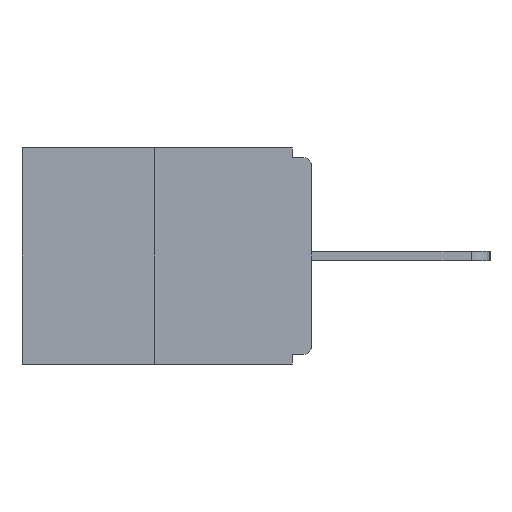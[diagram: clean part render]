
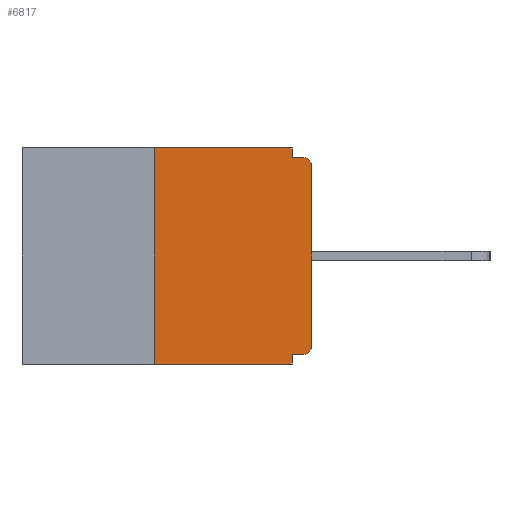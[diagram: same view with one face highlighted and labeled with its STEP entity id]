
A CAD part, left-side view. The second image highlights one B-rep face of the part: STEP entity #6817.
In plain terms, the highlighted planar face has unit normal (-1, 0, 0).
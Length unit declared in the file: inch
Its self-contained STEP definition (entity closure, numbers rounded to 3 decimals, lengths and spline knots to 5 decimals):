
#57 = DIRECTION ( 'NONE',  ( 0., 0., -1. ) ) ;
#111 = DIRECTION ( 'NONE',  ( 1., 0., 0. ) ) ;
#242 = EDGE_CURVE ( 'NONE', #7313, #13654, #5762, .T. ) ;
#287 = DIRECTION ( 'NONE',  ( 0., 0., -1. ) ) ;
#391 = CARTESIAN_POINT ( 'NONE',  ( 0., 0.031, 0. ) ) ;
#524 = DIRECTION ( 'NONE',  ( 0., 0., -1. ) ) ;
#777 = EDGE_CURVE ( 'NONE', #10795, #2583, #3986, .T. ) ;
#800 = DIRECTION ( 'NONE',  ( 0., -1., 0. ) ) ;
#875 = DIRECTION ( 'NONE',  ( -1., 0., 0. ) ) ;
#1165 = CARTESIAN_POINT ( 'NONE',  ( 0., 0.031, -0.328 ) ) ;
#1501 = DIRECTION ( 'NONE',  ( 0., 1., 0. ) ) ;
#1911 = CARTESIAN_POINT ( 'NONE',  ( 0., 0.031, -0.015 ) ) ;
#2117 = CARTESIAN_POINT ( 'NONE',  ( 0., 0.25, 0. ) ) ;
#2214 = CARTESIAN_POINT ( 'NONE',  ( 0., 0.46, 0. ) ) ;
#2464 = LINE ( 'NONE', #10610, #14768 ) ;
#2465 = LINE ( 'NONE', #13090, #2571 ) ;
#2571 = VECTOR ( 'NONE', #14127, 39.37008 ) ;
#2583 = VERTEX_POINT ( 'NONE', #1911 ) ;
#2786 = CARTESIAN_POINT ( 'NONE',  ( 0., 0.015, -0.015 ) ) ;
#2999 = VECTOR ( 'NONE', #13089, 39.37008 ) ;
#3040 = CARTESIAN_POINT ( 'NONE',  ( 0., 0.25, 0. ) ) ;
#3282 = FACE_OUTER_BOUND ( 'NONE', #11460, .T. ) ;
#3318 = AXIS2_PLACEMENT_3D ( 'NONE', #5569, #875, #57 ) ;
#3479 = EDGE_CURVE ( 'NONE', #9759, #9999, #5478, .T. ) ;
#3925 = LINE ( 'NONE', #10988, #14269 ) ;
#3986 = LINE ( 'NONE', #14268, #6601 ) ;
#4028 = DIRECTION ( 'NONE',  ( 0., 0., 1. ) ) ;
#4079 = AXIS2_PLACEMENT_3D ( 'NONE', #2214, #111, #11416 ) ;
#4212 = EDGE_CURVE ( 'NONE', #9239, #10795, #4382, .T. ) ;
#4382 = LINE ( 'NONE', #7358, #14359 ) ;
#4910 = EDGE_CURVE ( 'NONE', #10422, #6604, #2465, .T. ) ;
#5371 = ORIENTED_EDGE ( 'NONE', *, *, #3479, .T. ) ;
#5478 = CIRCLE ( 'NONE', #3318, 0.015 ) ;
#5569 = CARTESIAN_POINT ( 'NONE',  ( 0., 0.015, -0.313 ) ) ;
#5762 = CIRCLE ( 'NONE', #14151, 0.015 ) ;
#5909 = CARTESIAN_POINT ( 'NONE',  ( 0., 0., -0.03 ) ) ;
#6057 = ORIENTED_EDGE ( 'NONE', *, *, #242, .T. ) ;
#6298 = ORIENTED_EDGE ( 'NONE', *, *, #10361, .F. ) ;
#6601 = VECTOR ( 'NONE', #12259, 39.37008 ) ;
#6604 = VERTEX_POINT ( 'NONE', #12731 ) ;
#6817 = ADVANCED_FACE ( 'NONE', ( #3282 ), #7959, .F. ) ;
#6835 = VERTEX_POINT ( 'NONE', #1165 ) ;
#7279 = ORIENTED_EDGE ( 'NONE', *, *, #777, .F. ) ;
#7313 = VERTEX_POINT ( 'NONE', #5909 ) ;
#7329 = ORIENTED_EDGE ( 'NONE', *, *, #11288, .F. ) ;
#7358 = CARTESIAN_POINT ( 'NONE',  ( 0., 0.46, 0. ) ) ;
#7959 = PLANE ( 'NONE',  #4079 ) ;
#8171 = ORIENTED_EDGE ( 'NONE', *, *, #4910, .T. ) ;
#8285 = ORIENTED_EDGE ( 'NONE', *, *, #4212, .F. ) ;
#8504 = LINE ( 'NONE', #10829, #2999 ) ;
#8709 = ORIENTED_EDGE ( 'NONE', *, *, #12877, .T. ) ;
#9239 = VERTEX_POINT ( 'NONE', #2117 ) ;
#9723 = CARTESIAN_POINT ( 'NONE',  ( 0., 0.015, -0.03 ) ) ;
#9759 = VERTEX_POINT ( 'NONE', #12509 ) ;
#9999 = VERTEX_POINT ( 'NONE', #10217 ) ;
#10217 = CARTESIAN_POINT ( 'NONE',  ( 0., 0., -0.313 ) ) ;
#10361 = EDGE_CURVE ( 'NONE', #10422, #9239, #10731, .T. ) ;
#10422 = VERTEX_POINT ( 'NONE', #13719 ) ;
#10610 = CARTESIAN_POINT ( 'NONE',  ( 0., 0.031, -0.343 ) ) ;
#10731 = LINE ( 'NONE', #3040, #14704 ) ;
#10795 = VERTEX_POINT ( 'NONE', #391 ) ;
#10829 = CARTESIAN_POINT ( 'NONE',  ( 0., 0., 0. ) ) ;
#10988 = CARTESIAN_POINT ( 'NONE',  ( 0., 0., -0.328 ) ) ;
#11288 = EDGE_CURVE ( 'NONE', #2583, #13654, #14722, .T. ) ;
#11310 = DIRECTION ( 'NONE',  ( 0., -1., 0. ) ) ;
#11416 = DIRECTION ( 'NONE',  ( 0., 0., -1. ) ) ;
#11460 = EDGE_LOOP ( 'NONE', ( #8285, #6298, #8171, #12524, #13148, #5371, #8709, #6057, #7329, #7279 ) ) ;
#11985 = DIRECTION ( 'NONE',  ( -1., 0., 0. ) ) ;
#12259 = DIRECTION ( 'NONE',  ( 0., 0., -1. ) ) ;
#12406 = EDGE_CURVE ( 'NONE', #9759, #6835, #3925, .T. ) ;
#12509 = CARTESIAN_POINT ( 'NONE',  ( 0., 0.015, -0.328 ) ) ;
#12524 = ORIENTED_EDGE ( 'NONE', *, *, #12725, .F. ) ;
#12725 = EDGE_CURVE ( 'NONE', #6835, #6604, #2464, .T. ) ;
#12731 = CARTESIAN_POINT ( 'NONE',  ( 0., 0.031, -0.343 ) ) ;
#12877 = EDGE_CURVE ( 'NONE', #9999, #7313, #8504, .T. ) ;
#13089 = DIRECTION ( 'NONE',  ( 0., 0., 1. ) ) ;
#13090 = CARTESIAN_POINT ( 'NONE',  ( 0., 0.46, -0.343 ) ) ;
#13148 = ORIENTED_EDGE ( 'NONE', *, *, #12406, .F. ) ;
#13534 = CARTESIAN_POINT ( 'NONE',  ( 0., 0., -0.015 ) ) ;
#13544 = VECTOR ( 'NONE', #800, 39.37008 ) ;
#13654 = VERTEX_POINT ( 'NONE', #2786 ) ;
#13719 = CARTESIAN_POINT ( 'NONE',  ( 0., 0.25, -0.343 ) ) ;
#14127 = DIRECTION ( 'NONE',  ( 0., -1., 0. ) ) ;
#14151 = AXIS2_PLACEMENT_3D ( 'NONE', #9723, #11985, #524 ) ;
#14268 = CARTESIAN_POINT ( 'NONE',  ( 0., 0.031, 0. ) ) ;
#14269 = VECTOR ( 'NONE', #1501, 39.37008 ) ;
#14359 = VECTOR ( 'NONE', #11310, 39.37008 ) ;
#14704 = VECTOR ( 'NONE', #4028, 39.37008 ) ;
#14722 = LINE ( 'NONE', #13534, #13544 ) ;
#14768 = VECTOR ( 'NONE', #287, 39.37008 ) ;
